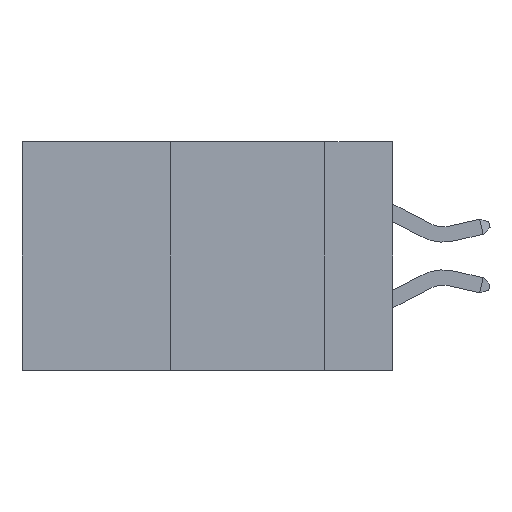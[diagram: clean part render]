
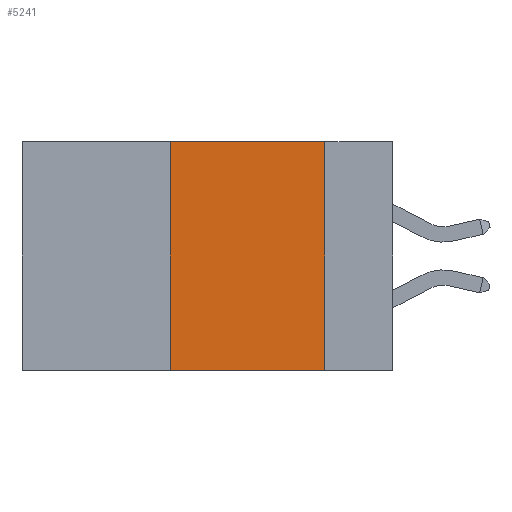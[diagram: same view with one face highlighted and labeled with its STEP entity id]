
A CAD part, left-side view. The second image highlights one B-rep face of the part: STEP entity #5241.
In plain terms, the highlighted planar face has unit normal (-1, 0, 0).
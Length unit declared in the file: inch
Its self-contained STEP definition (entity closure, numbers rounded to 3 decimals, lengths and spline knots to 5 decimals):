
#53 = ORIENTED_EDGE ( 'NONE', *, *, #2361, .F. ) ;
#231 = EDGE_CURVE ( 'NONE', #5583, #13741, #8226, .T. ) ;
#245 = DIRECTION ( 'NONE',  ( 0., 0., -1. ) ) ;
#542 = VECTOR ( 'NONE', #11905, 39.37008 ) ;
#1432 = CARTESIAN_POINT ( 'NONE',  ( 0., 0.6, 0. ) ) ;
#1642 = CARTESIAN_POINT ( 'NONE',  ( 0., 0.11, 0. ) ) ;
#2361 = EDGE_CURVE ( 'NONE', #3660, #7727, #3873, .T. ) ;
#2749 = DIRECTION ( 'NONE',  ( 0., -1., 0. ) ) ;
#2910 = CARTESIAN_POINT ( 'NONE',  ( 0., 0.6, 0. ) ) ;
#3282 = LINE ( 'NONE', #13901, #11102 ) ;
#3338 = CARTESIAN_POINT ( 'NONE',  ( 0., 0.36, 0. ) ) ;
#3660 = VERTEX_POINT ( 'NONE', #4180 ) ;
#3873 = LINE ( 'NONE', #1642, #7112 ) ;
#4180 = CARTESIAN_POINT ( 'NONE',  ( 0., 0.11, 0. ) ) ;
#5241 = ADVANCED_FACE ( 'NONE', ( #6767 ), #9129, .F. ) ;
#5580 = ORIENTED_EDGE ( 'NONE', *, *, #6601, .T. ) ;
#5583 = VERTEX_POINT ( 'NONE', #9674 ) ;
#6601 = EDGE_CURVE ( 'NONE', #5583, #7727, #3282, .T. ) ;
#6767 = FACE_OUTER_BOUND ( 'NONE', #9524, .T. ) ;
#7112 = VECTOR ( 'NONE', #13193, 39.37008 ) ;
#7727 = VERTEX_POINT ( 'NONE', #14308 ) ;
#8226 = LINE ( 'NONE', #11485, #13493 ) ;
#9129 = PLANE ( 'NONE',  #10937 ) ;
#9469 = DIRECTION ( 'NONE',  ( 0., 0., 1. ) ) ;
#9490 = ORIENTED_EDGE ( 'NONE', *, *, #9984, .F. ) ;
#9524 = EDGE_LOOP ( 'NONE', ( #53, #9490, #11552, #5580 ) ) ;
#9674 = CARTESIAN_POINT ( 'NONE',  ( 0., 0.36, -0.37 ) ) ;
#9984 = EDGE_CURVE ( 'NONE', #13741, #3660, #12191, .T. ) ;
#10937 = AXIS2_PLACEMENT_3D ( 'NONE', #1432, #11301, #245 ) ;
#11102 = VECTOR ( 'NONE', #2749, 39.37008 ) ;
#11301 = DIRECTION ( 'NONE',  ( 1., 0., 0. ) ) ;
#11485 = CARTESIAN_POINT ( 'NONE',  ( 0., 0.36, 0. ) ) ;
#11552 = ORIENTED_EDGE ( 'NONE', *, *, #231, .F. ) ;
#11905 = DIRECTION ( 'NONE',  ( 0., -1., 0. ) ) ;
#12191 = LINE ( 'NONE', #2910, #542 ) ;
#13193 = DIRECTION ( 'NONE',  ( 0., 0., -1. ) ) ;
#13493 = VECTOR ( 'NONE', #9469, 39.37008 ) ;
#13741 = VERTEX_POINT ( 'NONE', #3338 ) ;
#13901 = CARTESIAN_POINT ( 'NONE',  ( 0., 0.6, -0.37 ) ) ;
#14308 = CARTESIAN_POINT ( 'NONE',  ( 0., 0.11, -0.37 ) ) ;
